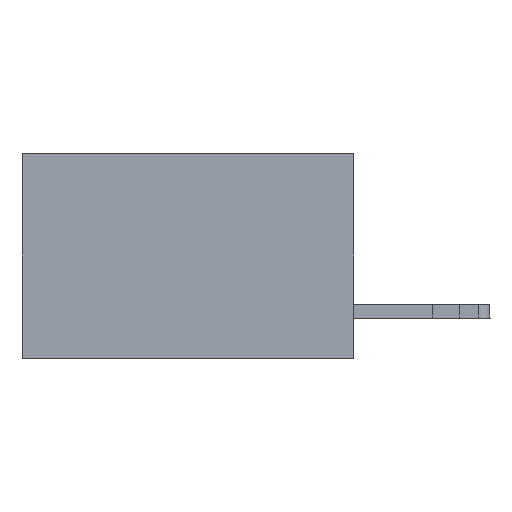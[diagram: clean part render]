
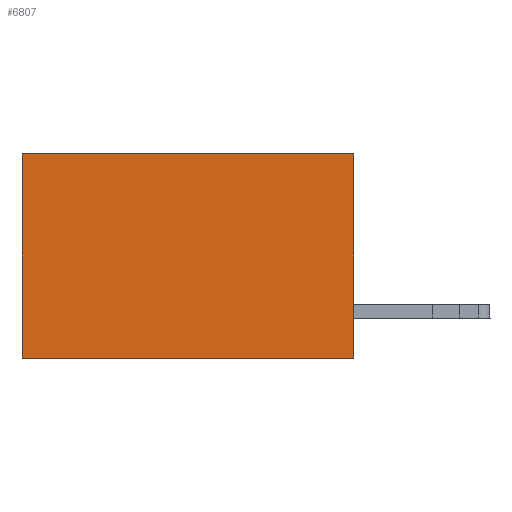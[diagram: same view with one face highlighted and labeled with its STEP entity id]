
A CAD part, left-side view. The second image highlights one B-rep face of the part: STEP entity #6807.
In plain terms, the highlighted planar face has unit normal (-1, 0, 0).
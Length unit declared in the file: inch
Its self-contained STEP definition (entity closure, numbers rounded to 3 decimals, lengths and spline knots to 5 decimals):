
#1363 = LINE ( 'NONE', #22754, #23644 ) ;
#2384 = DIRECTION ( 'NONE',  ( 0., 1., 0. ) ) ;
#2976 = LINE ( 'NONE', #39146, #26140 ) ;
#3161 = EDGE_CURVE ( 'NONE', #21676, #16401, #1363, .T. ) ;
#5156 = ORIENTED_EDGE ( 'NONE', *, *, #18891, .T. ) ;
#5519 = ORIENTED_EDGE ( 'NONE', *, *, #3161, .F. ) ;
#5667 = CARTESIAN_POINT ( 'NONE',  ( 0.2875, 0.6, 0. ) ) ;
#6807 = ADVANCED_FACE ( 'NONE', ( #10171 ), #34796, .F. ) ;
#10171 = FACE_OUTER_BOUND ( 'NONE', #23750, .T. ) ;
#12084 = VERTEX_POINT ( 'NONE', #19861 ) ;
#13861 = CARTESIAN_POINT ( 'NONE',  ( 0.2875, 0.6, -0.37 ) ) ;
#15514 = AXIS2_PLACEMENT_3D ( 'NONE', #19447, #27081, #39431 ) ;
#15979 = LINE ( 'NONE', #28272, #39509 ) ;
#16401 = VERTEX_POINT ( 'NONE', #13861 ) ;
#18065 = EDGE_CURVE ( 'NONE', #12084, #21676, #27100, .T. ) ;
#18606 = VERTEX_POINT ( 'NONE', #5667 ) ;
#18891 = EDGE_CURVE ( 'NONE', #12084, #18606, #2976, .T. ) ;
#19192 = DIRECTION ( 'NONE',  ( 0., 0., -1. ) ) ;
#19447 = CARTESIAN_POINT ( 'NONE',  ( 0.2875, 0., 0. ) ) ;
#19861 = CARTESIAN_POINT ( 'NONE',  ( 0.2875, 0., 0. ) ) ;
#20808 = CARTESIAN_POINT ( 'NONE',  ( 0.2875, 0., -0.37 ) ) ;
#20946 = ORIENTED_EDGE ( 'NONE', *, *, #37303, .T. ) ;
#21370 = VECTOR ( 'NONE', #24246, 39.37008 ) ;
#21638 = CARTESIAN_POINT ( 'NONE',  ( 0.2875, 0., 0. ) ) ;
#21676 = VERTEX_POINT ( 'NONE', #20808 ) ;
#22754 = CARTESIAN_POINT ( 'NONE',  ( 0.2875, 0., -0.37 ) ) ;
#23644 = VECTOR ( 'NONE', #32260, 39.37008 ) ;
#23750 = EDGE_LOOP ( 'NONE', ( #20946, #5519, #24492, #5156 ) ) ;
#24246 = DIRECTION ( 'NONE',  ( 0., 0., -1. ) ) ;
#24492 = ORIENTED_EDGE ( 'NONE', *, *, #18065, .F. ) ;
#26140 = VECTOR ( 'NONE', #2384, 39.37008 ) ;
#27081 = DIRECTION ( 'NONE',  ( 1., 0., 0. ) ) ;
#27100 = LINE ( 'NONE', #21638, #21370 ) ;
#28272 = CARTESIAN_POINT ( 'NONE',  ( 0.2875, 0.6, 0. ) ) ;
#32260 = DIRECTION ( 'NONE',  ( 0., 1., 0. ) ) ;
#34796 = PLANE ( 'NONE',  #15514 ) ;
#37303 = EDGE_CURVE ( 'NONE', #18606, #16401, #15979, .T. ) ;
#39146 = CARTESIAN_POINT ( 'NONE',  ( 0.2875, 0., 0. ) ) ;
#39431 = DIRECTION ( 'NONE',  ( 0., 0., -1. ) ) ;
#39509 = VECTOR ( 'NONE', #19192, 39.37008 ) ;
